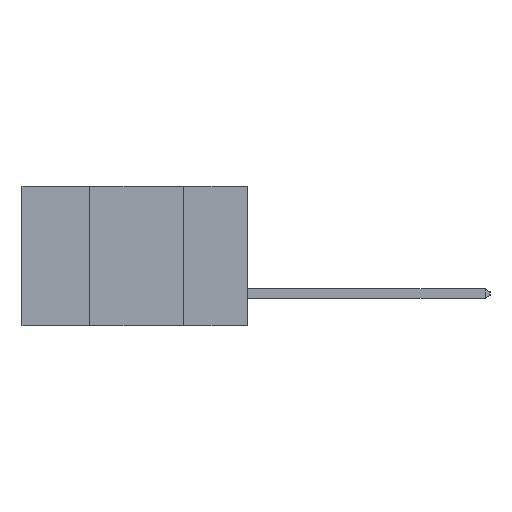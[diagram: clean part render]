
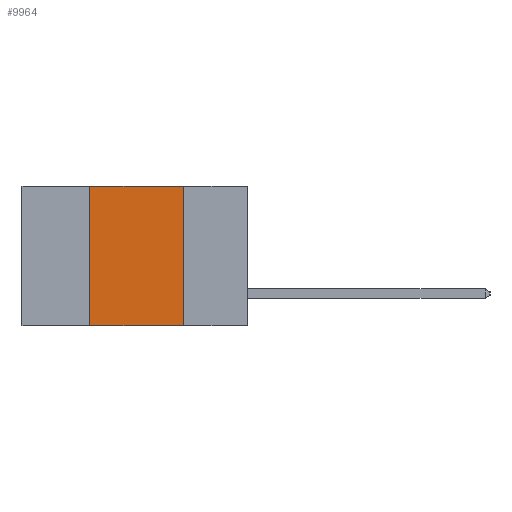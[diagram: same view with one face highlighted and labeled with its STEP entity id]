
A CAD part, left-side view. The second image highlights one B-rep face of the part: STEP entity #9964.
In plain terms, the highlighted planar face has unit normal (-1, 0, 0).
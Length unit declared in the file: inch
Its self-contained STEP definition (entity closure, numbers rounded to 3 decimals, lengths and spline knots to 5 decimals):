
#185 = EDGE_CURVE ( 'NONE', #9841, #10042, #1633, .T. ) ;
#420 = ORIENTED_EDGE ( 'NONE', *, *, #6430, .F. ) ;
#450 = ORIENTED_EDGE ( 'NONE', *, *, #3940, .F. ) ;
#570 = ORIENTED_EDGE ( 'NONE', *, *, #8292, .F. ) ;
#633 = ORIENTED_EDGE ( 'NONE', *, *, #185, .T. ) ;
#1102 = AXIS2_PLACEMENT_3D ( 'NONE', #7850, #4645, #10181 ) ;
#1633 = LINE ( 'NONE', #1922, #5728 ) ;
#1893 = DIRECTION ( 'NONE',  ( 0., -1., 0. ) ) ;
#1922 = CARTESIAN_POINT ( 'NONE',  ( 0., 0.6, -0.37 ) ) ;
#2582 = CARTESIAN_POINT ( 'NONE',  ( 0., 0.6, 0. ) ) ;
#3132 = LINE ( 'NONE', #7548, #6916 ) ;
#3195 = DIRECTION ( 'NONE',  ( 0., -1., 0. ) ) ;
#3940 = EDGE_CURVE ( 'NONE', #6130, #10009, #4420, .T. ) ;
#4420 = LINE ( 'NONE', #2582, #8176 ) ;
#4645 = DIRECTION ( 'NONE',  ( 1., 0., 0. ) ) ;
#5728 = VECTOR ( 'NONE', #1893, 39.37008 ) ;
#6118 = CARTESIAN_POINT ( 'NONE',  ( 0., 0.42, -0.37 ) ) ;
#6130 = VERTEX_POINT ( 'NONE', #8652 ) ;
#6133 = VECTOR ( 'NONE', #8181, 39.37008 ) ;
#6430 = EDGE_CURVE ( 'NONE', #10009, #10042, #3132, .T. ) ;
#6916 = VECTOR ( 'NONE', #7500, 39.37008 ) ;
#7125 = CARTESIAN_POINT ( 'NONE',  ( 0., 0.17, 0. ) ) ;
#7478 = EDGE_LOOP ( 'NONE', ( #420, #450, #570, #633 ) ) ;
#7500 = DIRECTION ( 'NONE',  ( 0., 0., -1. ) ) ;
#7548 = CARTESIAN_POINT ( 'NONE',  ( 0., 0.17, 0. ) ) ;
#7850 = CARTESIAN_POINT ( 'NONE',  ( 0., 0.6, 0. ) ) ;
#8176 = VECTOR ( 'NONE', #3195, 39.37008 ) ;
#8181 = DIRECTION ( 'NONE',  ( 0., 0., 1. ) ) ;
#8287 = CARTESIAN_POINT ( 'NONE',  ( 0., 0.42, 0. ) ) ;
#8292 = EDGE_CURVE ( 'NONE', #9841, #6130, #8500, .T. ) ;
#8500 = LINE ( 'NONE', #8287, #6133 ) ;
#8652 = CARTESIAN_POINT ( 'NONE',  ( 0., 0.42, 0. ) ) ;
#8725 = CARTESIAN_POINT ( 'NONE',  ( 0., 0.17, -0.37 ) ) ;
#9430 = PLANE ( 'NONE',  #1102 ) ;
#9841 = VERTEX_POINT ( 'NONE', #6118 ) ;
#9964 = ADVANCED_FACE ( 'NONE', ( #10378 ), #9430, .F. ) ;
#10009 = VERTEX_POINT ( 'NONE', #7125 ) ;
#10042 = VERTEX_POINT ( 'NONE', #8725 ) ;
#10181 = DIRECTION ( 'NONE',  ( 0., 0., -1. ) ) ;
#10378 = FACE_OUTER_BOUND ( 'NONE', #7478, .T. ) ;
